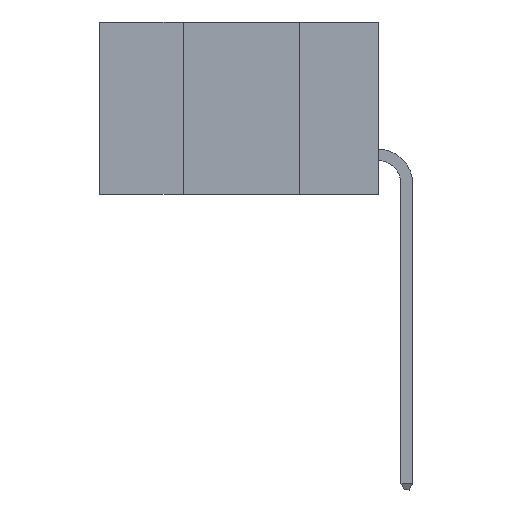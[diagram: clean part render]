
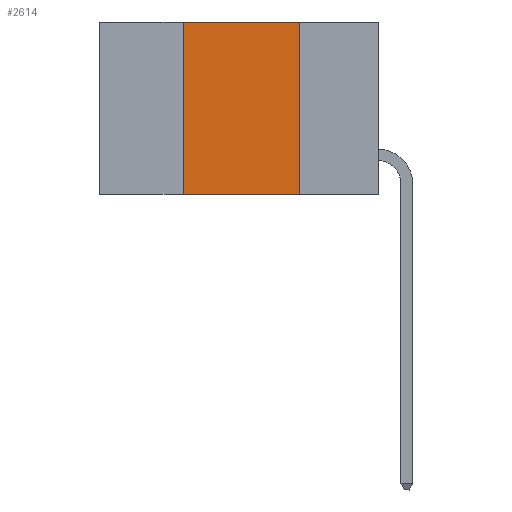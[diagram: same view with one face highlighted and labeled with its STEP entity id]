
A CAD part, left-side view. The second image highlights one B-rep face of the part: STEP entity #2614.
In plain terms, the highlighted planar face has unit normal (-1, 0, 0).
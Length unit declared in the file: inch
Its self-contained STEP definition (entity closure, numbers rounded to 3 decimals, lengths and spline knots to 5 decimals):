
#169 = VERTEX_POINT ( 'NONE', #343 ) ;
#343 = CARTESIAN_POINT ( 'NONE',  ( 0., 0.17, 0. ) ) ;
#533 = ORIENTED_EDGE ( 'NONE', *, *, #3300, .F. ) ;
#654 = CARTESIAN_POINT ( 'NONE',  ( 0., 0.42, 0. ) ) ;
#1658 = DIRECTION ( 'NONE',  ( 0., -1., 0. ) ) ;
#1816 = DIRECTION ( 'NONE',  ( 0., 0., 1. ) ) ;
#2254 = CARTESIAN_POINT ( 'NONE',  ( 0., 0.42, 0. ) ) ;
#2265 = CARTESIAN_POINT ( 'NONE',  ( 0., 0.17, -0.37 ) ) ;
#2417 = VECTOR ( 'NONE', #10146, 39.37008 ) ;
#2614 = ADVANCED_FACE ( 'NONE', ( #8254 ), #10912, .F. ) ;
#2692 = ORIENTED_EDGE ( 'NONE', *, *, #6689, .T. ) ;
#2847 = CARTESIAN_POINT ( 'NONE',  ( 0., 0.17, 0. ) ) ;
#3172 = LINE ( 'NONE', #654, #8391 ) ;
#3300 = EDGE_CURVE ( 'NONE', #11256, #169, #5484, .T. ) ;
#3412 = ORIENTED_EDGE ( 'NONE', *, *, #10908, .F. ) ;
#3790 = AXIS2_PLACEMENT_3D ( 'NONE', #8215, #12346, #7922 ) ;
#5376 = VECTOR ( 'NONE', #1658, 39.37008 ) ;
#5484 = LINE ( 'NONE', #8658, #13575 ) ;
#6392 = ORIENTED_EDGE ( 'NONE', *, *, #8120, .F. ) ;
#6689 = EDGE_CURVE ( 'NONE', #7067, #8382, #13184, .T. ) ;
#7067 = VERTEX_POINT ( 'NONE', #12666 ) ;
#7524 = EDGE_LOOP ( 'NONE', ( #3412, #533, #6392, #2692 ) ) ;
#7922 = DIRECTION ( 'NONE',  ( 0., 0., -1. ) ) ;
#8001 = LINE ( 'NONE', #2847, #2417 ) ;
#8120 = EDGE_CURVE ( 'NONE', #7067, #11256, #3172, .T. ) ;
#8215 = CARTESIAN_POINT ( 'NONE',  ( 0., 0.6, 0. ) ) ;
#8254 = FACE_OUTER_BOUND ( 'NONE', #7524, .T. ) ;
#8382 = VERTEX_POINT ( 'NONE', #2265 ) ;
#8391 = VECTOR ( 'NONE', #1816, 39.37008 ) ;
#8658 = CARTESIAN_POINT ( 'NONE',  ( 0., 0.6, 0. ) ) ;
#10146 = DIRECTION ( 'NONE',  ( 0., 0., -1. ) ) ;
#10908 = EDGE_CURVE ( 'NONE', #169, #8382, #8001, .T. ) ;
#10912 = PLANE ( 'NONE',  #3790 ) ;
#11256 = VERTEX_POINT ( 'NONE', #2254 ) ;
#12121 = CARTESIAN_POINT ( 'NONE',  ( 0., 0.6, -0.37 ) ) ;
#12346 = DIRECTION ( 'NONE',  ( 1., 0., 0. ) ) ;
#12666 = CARTESIAN_POINT ( 'NONE',  ( 0., 0.42, -0.37 ) ) ;
#12695 = DIRECTION ( 'NONE',  ( 0., -1., 0. ) ) ;
#13184 = LINE ( 'NONE', #12121, #5376 ) ;
#13575 = VECTOR ( 'NONE', #12695, 39.37008 ) ;
